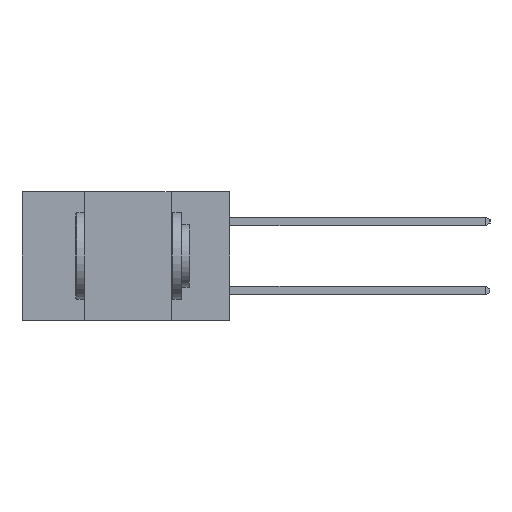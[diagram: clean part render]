
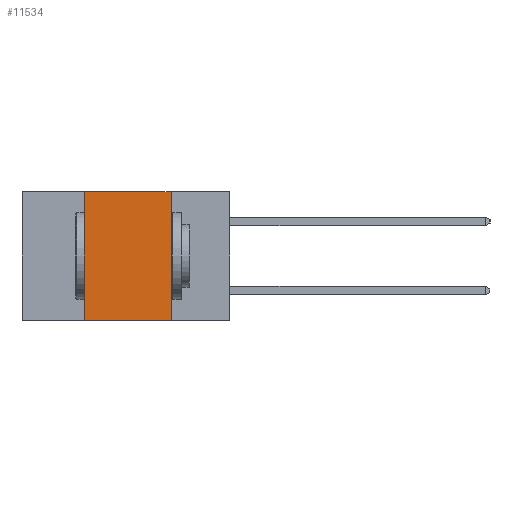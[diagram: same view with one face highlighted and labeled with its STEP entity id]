
A CAD part, left-side view. The second image highlights one B-rep face of the part: STEP entity #11534.
In plain terms, the highlighted planar face has unit normal (-1, 0, 0).
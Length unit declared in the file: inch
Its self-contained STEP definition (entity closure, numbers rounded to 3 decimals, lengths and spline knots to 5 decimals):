
#83 = EDGE_LOOP ( 'NONE', ( #4405, #10058, #12508, #280 ) ) ;
#158 = DIRECTION ( 'NONE',  ( 0., 0., -1. ) ) ;
#233 = LINE ( 'NONE', #7253, #7849 ) ;
#280 = ORIENTED_EDGE ( 'NONE', *, *, #7060, .T. ) ;
#759 = CARTESIAN_POINT ( 'NONE',  ( 0., 0.17, -0.37 ) ) ;
#1156 = EDGE_CURVE ( 'NONE', #3792, #9047, #1944, .T. ) ;
#1650 = CARTESIAN_POINT ( 'NONE',  ( 0., 0.6, 0. ) ) ;
#1773 = VERTEX_POINT ( 'NONE', #8529 ) ;
#1868 = CARTESIAN_POINT ( 'NONE',  ( 0., 0.17, 0. ) ) ;
#1944 = LINE ( 'NONE', #1650, #6892 ) ;
#2549 = VERTEX_POINT ( 'NONE', #759 ) ;
#2850 = EDGE_CURVE ( 'NONE', #9047, #2549, #9660, .T. ) ;
#3002 = FACE_OUTER_BOUND ( 'NONE', #83, .T. ) ;
#3027 = CARTESIAN_POINT ( 'NONE',  ( 0., 0.42, 0. ) ) ;
#3792 = VERTEX_POINT ( 'NONE', #7797 ) ;
#4375 = CARTESIAN_POINT ( 'NONE',  ( 0., 0.6, 0. ) ) ;
#4405 = ORIENTED_EDGE ( 'NONE', *, *, #2850, .F. ) ;
#5355 = DIRECTION ( 'NONE',  ( 0., 0., -1. ) ) ;
#5465 = AXIS2_PLACEMENT_3D ( 'NONE', #4375, #11003, #5355 ) ;
#6844 = DIRECTION ( 'NONE',  ( 0., -1., 0. ) ) ;
#6892 = VECTOR ( 'NONE', #11945, 39.37008 ) ;
#7060 = EDGE_CURVE ( 'NONE', #1773, #2549, #233, .T. ) ;
#7253 = CARTESIAN_POINT ( 'NONE',  ( 0., 0.6, -0.37 ) ) ;
#7797 = CARTESIAN_POINT ( 'NONE',  ( 0., 0.42, 0. ) ) ;
#7849 = VECTOR ( 'NONE', #6844, 39.37008 ) ;
#8084 = VECTOR ( 'NONE', #8832, 39.37008 ) ;
#8529 = CARTESIAN_POINT ( 'NONE',  ( 0., 0.42, -0.37 ) ) ;
#8832 = DIRECTION ( 'NONE',  ( 0., 0., 1. ) ) ;
#9047 = VERTEX_POINT ( 'NONE', #12113 ) ;
#9660 = LINE ( 'NONE', #1868, #11825 ) ;
#9957 = EDGE_CURVE ( 'NONE', #1773, #3792, #11129, .T. ) ;
#10058 = ORIENTED_EDGE ( 'NONE', *, *, #1156, .F. ) ;
#10067 = PLANE ( 'NONE',  #5465 ) ;
#11003 = DIRECTION ( 'NONE',  ( 1., 0., 0. ) ) ;
#11129 = LINE ( 'NONE', #3027, #8084 ) ;
#11534 = ADVANCED_FACE ( 'NONE', ( #3002 ), #10067, .F. ) ;
#11825 = VECTOR ( 'NONE', #158, 39.37008 ) ;
#11945 = DIRECTION ( 'NONE',  ( 0., -1., 0. ) ) ;
#12113 = CARTESIAN_POINT ( 'NONE',  ( 0., 0.17, 0. ) ) ;
#12508 = ORIENTED_EDGE ( 'NONE', *, *, #9957, .F. ) ;
